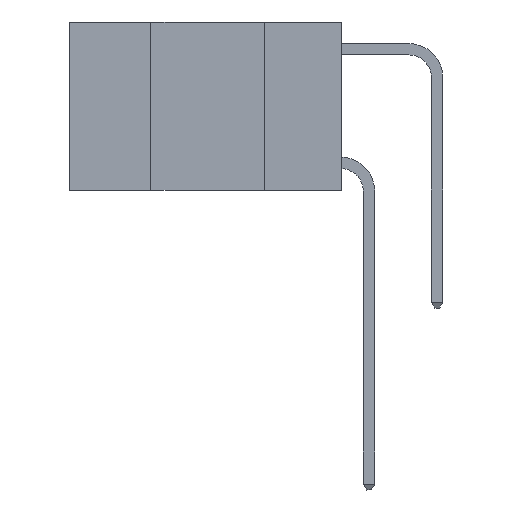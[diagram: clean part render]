
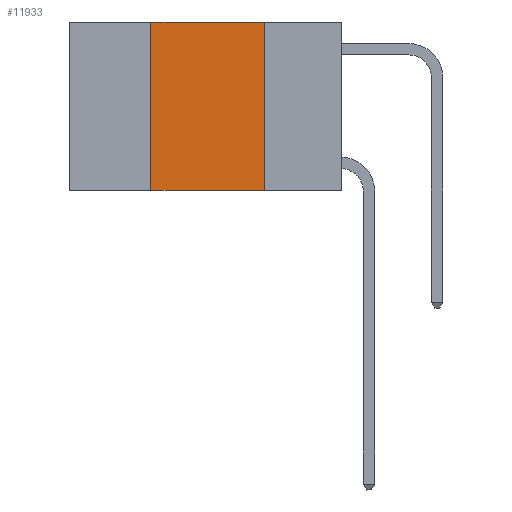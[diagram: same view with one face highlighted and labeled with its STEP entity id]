
A CAD part, left-side view. The second image highlights one B-rep face of the part: STEP entity #11933.
In plain terms, the highlighted planar face has unit normal (-1, 0, 0).
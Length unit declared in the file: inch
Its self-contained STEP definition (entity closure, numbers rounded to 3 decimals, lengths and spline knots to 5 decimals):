
#582 = VECTOR ( 'NONE', #9462, 39.37008 ) ;
#1112 = VECTOR ( 'NONE', #4877, 39.37008 ) ;
#1121 = VECTOR ( 'NONE', #4008, 39.37008 ) ;
#1292 = CARTESIAN_POINT ( 'NONE',  ( 0., 0.42, 0. ) ) ;
#1371 = CARTESIAN_POINT ( 'NONE',  ( 0., 0.17, 0. ) ) ;
#1590 = ORIENTED_EDGE ( 'NONE', *, *, #13792, .F. ) ;
#1939 = EDGE_LOOP ( 'NONE', ( #13036, #3231, #1590, #6645 ) ) ;
#2276 = EDGE_CURVE ( 'NONE', #8932, #12706, #6295, .T. ) ;
#2649 = EDGE_CURVE ( 'NONE', #12345, #12706, #3018, .T. ) ;
#3018 = LINE ( 'NONE', #8224, #7940 ) ;
#3231 = ORIENTED_EDGE ( 'NONE', *, *, #6835, .F. ) ;
#4008 = DIRECTION ( 'NONE',  ( 0., 0., -1. ) ) ;
#4133 = DIRECTION ( 'NONE',  ( 0., 0., -1. ) ) ;
#4877 = DIRECTION ( 'NONE',  ( 0., 0., 1. ) ) ;
#5087 = LINE ( 'NONE', #10200, #1112 ) ;
#5094 = CARTESIAN_POINT ( 'NONE',  ( 0., 0.6, 0. ) ) ;
#5241 = CARTESIAN_POINT ( 'NONE',  ( 0., 0.42, -0.37 ) ) ;
#5255 = PLANE ( 'NONE',  #10938 ) ;
#6295 = LINE ( 'NONE', #11491, #1121 ) ;
#6410 = DIRECTION ( 'NONE',  ( 1., 0., 0. ) ) ;
#6645 = ORIENTED_EDGE ( 'NONE', *, *, #2649, .T. ) ;
#6835 = EDGE_CURVE ( 'NONE', #12624, #8932, #12446, .T. ) ;
#7940 = VECTOR ( 'NONE', #9347, 39.37008 ) ;
#8224 = CARTESIAN_POINT ( 'NONE',  ( 0., 0.6, -0.37 ) ) ;
#8932 = VERTEX_POINT ( 'NONE', #1371 ) ;
#9347 = DIRECTION ( 'NONE',  ( 0., -1., 0. ) ) ;
#9462 = DIRECTION ( 'NONE',  ( 0., -1., 0. ) ) ;
#10200 = CARTESIAN_POINT ( 'NONE',  ( 0., 0.42, 0. ) ) ;
#10518 = CARTESIAN_POINT ( 'NONE',  ( 0., 0.6, 0. ) ) ;
#10938 = AXIS2_PLACEMENT_3D ( 'NONE', #10518, #6410, #4133 ) ;
#11491 = CARTESIAN_POINT ( 'NONE',  ( 0., 0.17, 0. ) ) ;
#11838 = CARTESIAN_POINT ( 'NONE',  ( 0., 0.17, -0.37 ) ) ;
#11910 = FACE_OUTER_BOUND ( 'NONE', #1939, .T. ) ;
#11933 = ADVANCED_FACE ( 'NONE', ( #11910 ), #5255, .F. ) ;
#12345 = VERTEX_POINT ( 'NONE', #5241 ) ;
#12446 = LINE ( 'NONE', #5094, #582 ) ;
#12624 = VERTEX_POINT ( 'NONE', #1292 ) ;
#12706 = VERTEX_POINT ( 'NONE', #11838 ) ;
#13036 = ORIENTED_EDGE ( 'NONE', *, *, #2276, .F. ) ;
#13792 = EDGE_CURVE ( 'NONE', #12345, #12624, #5087, .T. ) ;
